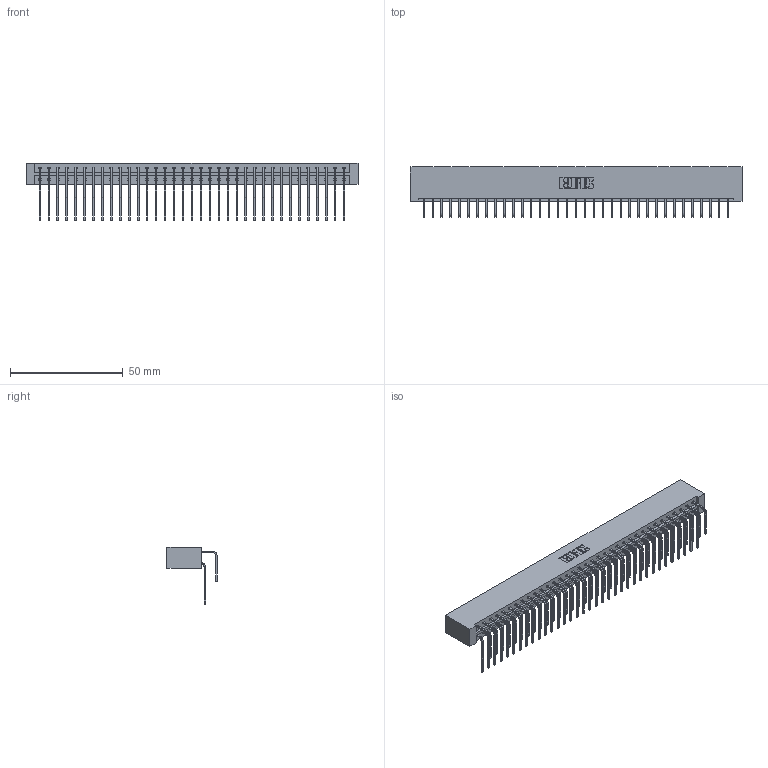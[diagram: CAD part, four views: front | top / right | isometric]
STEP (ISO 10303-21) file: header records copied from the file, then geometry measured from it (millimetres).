
FILE_DESCRIPTION (( 'STEP AP203' ), '1' );
FILE_NAME ('333-070-558-201.STEP', '2018-08-04T15:27:36', ( '' ), ( '' ), 'SwSTEP 2.0', 'SolidWorks 2016', '' );
FILE_SCHEMA (( 'CONFIG_CONTROL_DESIGN' ));
Length unit declared in the file: inch
Products named in the file (4): 333 Part_Lugless; 345-292-001_558 559 Tail - 1; 345-292-001_558 Tail - 2; 333-070-558-201
Assembly tree (71 placements, depth 2):
  333-070-558-201
    333 Part_Lugless
    345-292-001_558 559 Tail - 1  x35
    345-292-001_558 Tail - 2  x35
Bounding box: 146.94 x 22.17 x 25.53 mm (x, y, z)
Volume: 15972.2 mm3; surface area: 20843.7 mm2
Topology: 71 solids, 71 shells, 3886 faces, 11557 edges, 7610 vertices
Faces by surface type: plane 2726, cylinder 1160
Entity records: 24929 total; most frequent: CARTESIAN_POINT 4189, ORIENTED_EDGE 4074, DIRECTION 3565, EDGE_CURVE 2037, LINE 1877, VECTOR 1877, VERTEX_POINT 1354, AXIS2_PLACEMENT_3D 844
